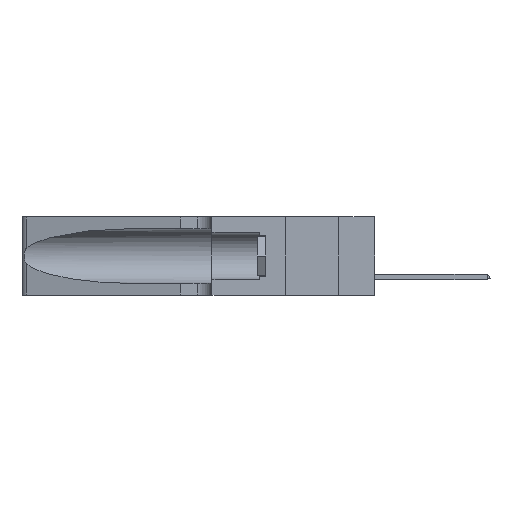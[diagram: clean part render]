
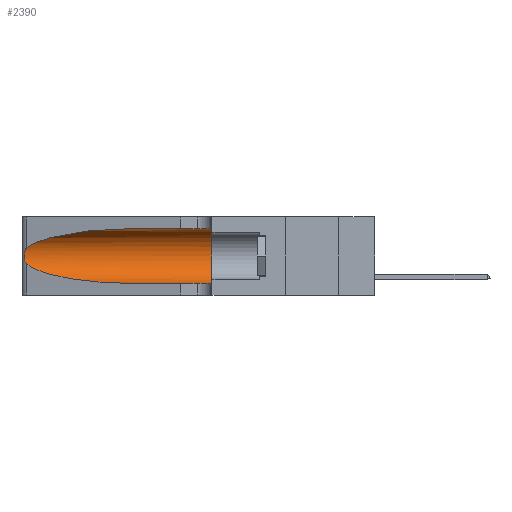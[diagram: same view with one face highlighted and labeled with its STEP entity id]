
A CAD part, left-side view. The second image highlights one B-rep face of the part: STEP entity #2390.
In plain terms, the highlighted cylindrical face has radius 3.308 mm (diameter 6.617 mm), a partial arc.
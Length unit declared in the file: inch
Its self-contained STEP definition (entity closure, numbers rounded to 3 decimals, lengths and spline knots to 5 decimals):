
#139 = CARTESIAN_POINT ( 'NONE',  ( 0.1305, 0.72297, 0.31525 ) ) ;
#249 = CARTESIAN_POINT ( 'NONE',  ( 0.18966, 0.96281, 0.05475 ) ) ;
#394 = CARTESIAN_POINT ( 'NONE',  ( 0.25787, 1.23484, 0.2124 ) ) ;
#823 =( BOUNDED_CURVE ( )  B_SPLINE_CURVE ( 3, ( #17930, #18088, #5320, #5404 ),
 .UNSPECIFIED., .F., .T. ) 
 B_SPLINE_CURVE_WITH_KNOTS ( ( 4, 4 ),
 ( 1.5708, 2.84003 ),
 .UNSPECIFIED. ) 
 CURVE ( )  GEOMETRIC_REPRESENTATION_ITEM ( )  RATIONAL_B_SPLINE_CURVE ( ( 1., 0.87, 0.87, 1. ) ) 
 REPRESENTATION_ITEM ( '' )  );
#1230 = CARTESIAN_POINT ( 'NONE',  ( 0.25639, 1.23186, 0.15144 ) ) ;
#2390 = ADVANCED_FACE ( 'NONE', ( #9756 ), #18517, .F. ) ;
#2705 = CARTESIAN_POINT ( 'NONE',  ( 0.25487, 1.22718, 0.22369 ) ) ;
#2755 = ORIENTED_EDGE ( 'NONE', *, *, #8996, .T. ) ;
#3034 = DIRECTION ( 'NONE',  ( 0., 1., 0. ) ) ;
#3283 =( BOUNDED_CURVE ( )  B_SPLINE_CURVE ( 3, ( #13023, #13188, #249, #7762 ),
 .UNSPECIFIED., .F., .F. ) 
 B_SPLINE_CURVE_WITH_KNOTS ( ( 4, 4 ),
 ( 3.44316, 4.71239 ),
 .UNSPECIFIED. ) 
 CURVE ( )  GEOMETRIC_REPRESENTATION_ITEM ( )  RATIONAL_B_SPLINE_CURVE ( ( 1., 0.87, 0.87, 1. ) ) 
 REPRESENTATION_ITEM ( '' )  );
#3586 = B_SPLINE_CURVE_WITH_KNOTS ( 'NONE', 3,
 ( #16484, #5668, #5782, #394, #20563, #5859, #11442, #18728, #9720, #7875, #19496, #1230, #13995, #23111 ),
 .UNSPECIFIED., .F., .F.,
 ( 4, 2, 2, 2, 2, 2, 4 ),
 ( 0., 0.00027, 0.00053, 0.00107, 0.0016, 0.00187, 0.00214 ),
 .UNSPECIFIED. ) ;
#3740 = VERTEX_POINT ( 'NONE', #5577 ) ;
#4173 = EDGE_CURVE ( 'NONE', #16101, #23296, #823, .T. ) ;
#4194 = CARTESIAN_POINT ( 'NONE',  ( 0.1305, 1.61858, 0.31525 ) ) ;
#4459 = ORIENTED_EDGE ( 'NONE', *, *, #16232, .F. ) ;
#4603 = DIRECTION ( 'NONE',  ( 0., 0., 1. ) ) ;
#4733 = ORIENTED_EDGE ( 'NONE', *, *, #4173, .T. ) ;
#5320 = CARTESIAN_POINT ( 'NONE',  ( 0.2373, 1.15595, 0.28018 ) ) ;
#5402 = CIRCLE ( 'NONE', #7703, 0.13025 ) ;
#5404 = CARTESIAN_POINT ( 'NONE',  ( 0.25487, 1.22718, 0.22369 ) ) ;
#5577 = CARTESIAN_POINT ( 'NONE',  ( 0.1305, 0.35, 0.31525 ) ) ;
#5668 = CARTESIAN_POINT ( 'NONE',  ( 0.25555, 1.22994, 0.2215 ) ) ;
#5669 = CARTESIAN_POINT ( 'NONE',  ( 0.1305, 1.61858, 0.185 ) ) ;
#5782 = CARTESIAN_POINT ( 'NONE',  ( 0.25639, 1.23184, 0.21858 ) ) ;
#5859 = CARTESIAN_POINT ( 'NONE',  ( 0.26018, 1.23835, 0.19895 ) ) ;
#6146 = EDGE_CURVE ( 'NONE', #23296, #10497, #3586, .T. ) ;
#7063 = EDGE_CURVE ( 'NONE', #12615, #16260, #18894, .T. ) ;
#7640 = DIRECTION ( 'NONE',  ( 0., -1., 0. ) ) ;
#7703 = AXIS2_PLACEMENT_3D ( 'NONE', #22708, #3034, #4603 ) ;
#7762 = CARTESIAN_POINT ( 'NONE',  ( 0.1305, 0.72297, 0.05475 ) ) ;
#7875 = CARTESIAN_POINT ( 'NONE',  ( 0.25856, 1.23593, 0.16098 ) ) ;
#8996 = EDGE_CURVE ( 'NONE', #10497, #12615, #3283, .T. ) ;
#9530 = DIRECTION ( 'NONE',  ( 0., 0., -1. ) ) ;
#9720 = CARTESIAN_POINT ( 'NONE',  ( 0.26017, 1.23833, 0.17102 ) ) ;
#9756 = FACE_OUTER_BOUND ( 'NONE', #16982, .T. ) ;
#10286 = AXIS2_PLACEMENT_3D ( 'NONE', #5669, #13055, #9530 ) ;
#10497 = VERTEX_POINT ( 'NONE', #20412 ) ;
#11442 = CARTESIAN_POINT ( 'NONE',  ( 0.26075, 1.23896, 0.19203 ) ) ;
#12615 = VERTEX_POINT ( 'NONE', #16158 ) ;
#13023 = CARTESIAN_POINT ( 'NONE',  ( 0.25487, 1.22718, 0.14631 ) ) ;
#13055 = DIRECTION ( 'NONE',  ( 0., -1., 0. ) ) ;
#13188 = CARTESIAN_POINT ( 'NONE',  ( 0.2373, 1.15595, 0.08982 ) ) ;
#13905 = LINE ( 'NONE', #4194, #18149 ) ;
#13995 = CARTESIAN_POINT ( 'NONE',  ( 0.25555, 1.22993, 0.14849 ) ) ;
#15741 = ORIENTED_EDGE ( 'NONE', *, *, #6146, .T. ) ;
#15767 = VECTOR ( 'NONE', #7640, 39.37008 ) ;
#16074 = DIRECTION ( 'NONE',  ( 0., -1., 0. ) ) ;
#16101 = VERTEX_POINT ( 'NONE', #139 ) ;
#16158 = CARTESIAN_POINT ( 'NONE',  ( 0.1305, 0.72297, 0.05475 ) ) ;
#16232 = EDGE_CURVE ( 'NONE', #16101, #3740, #13905, .T. ) ;
#16260 = VERTEX_POINT ( 'NONE', #19603 ) ;
#16484 = CARTESIAN_POINT ( 'NONE',  ( 0.25487, 1.22718, 0.22369 ) ) ;
#16982 = EDGE_LOOP ( 'NONE', ( #4733, #15741, #2755, #21248, #22987, #4459 ) ) ;
#17930 = CARTESIAN_POINT ( 'NONE',  ( 0.1305, 0.72297, 0.31525 ) ) ;
#18088 = CARTESIAN_POINT ( 'NONE',  ( 0.18966, 0.96281, 0.31525 ) ) ;
#18149 = VECTOR ( 'NONE', #16074, 39.37008 ) ;
#18517 = CYLINDRICAL_SURFACE ( 'NONE', #10286, 0.13025 ) ;
#18728 = CARTESIAN_POINT ( 'NONE',  ( 0.26075, 1.23896, 0.178 ) ) ;
#18894 = LINE ( 'NONE', #20053, #15767 ) ;
#19496 = CARTESIAN_POINT ( 'NONE',  ( 0.25789, 1.23486, 0.15765 ) ) ;
#19603 = CARTESIAN_POINT ( 'NONE',  ( 0.1305, 0.35, 0.05475 ) ) ;
#20053 = CARTESIAN_POINT ( 'NONE',  ( 0.1305, 1.61858, 0.05475 ) ) ;
#20412 = CARTESIAN_POINT ( 'NONE',  ( 0.25487, 1.22718, 0.14631 ) ) ;
#20563 = CARTESIAN_POINT ( 'NONE',  ( 0.25854, 1.2359, 0.20912 ) ) ;
#20618 = EDGE_CURVE ( 'NONE', #3740, #16260, #5402, .T. ) ;
#21248 = ORIENTED_EDGE ( 'NONE', *, *, #7063, .T. ) ;
#22708 = CARTESIAN_POINT ( 'NONE',  ( 0.1305, 0.35, 0.185 ) ) ;
#22987 = ORIENTED_EDGE ( 'NONE', *, *, #20618, .F. ) ;
#23111 = CARTESIAN_POINT ( 'NONE',  ( 0.25487, 1.22718, 0.14631 ) ) ;
#23296 = VERTEX_POINT ( 'NONE', #2705 ) ;
